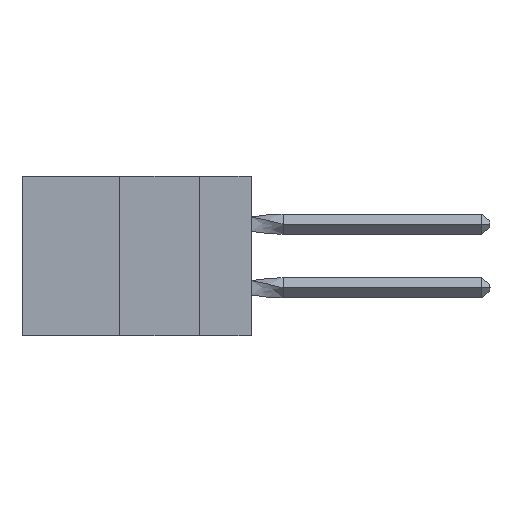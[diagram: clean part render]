
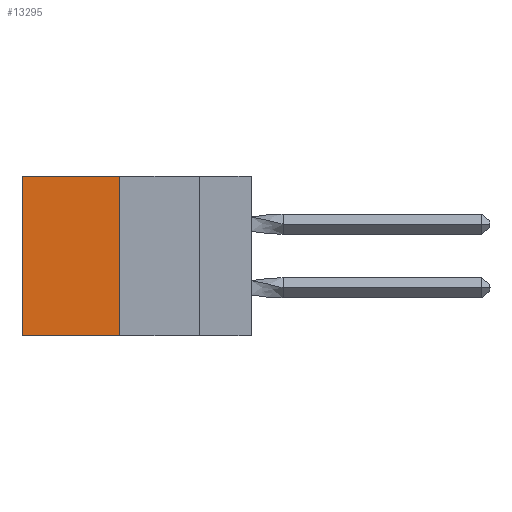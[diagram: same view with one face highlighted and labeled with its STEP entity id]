
A CAD part, left-side view. The second image highlights one B-rep face of the part: STEP entity #13295.
In plain terms, the highlighted planar face has unit normal (-1, 0, 0).
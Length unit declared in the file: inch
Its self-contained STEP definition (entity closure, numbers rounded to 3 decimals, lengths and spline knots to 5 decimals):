
#502 = CARTESIAN_POINT ( 'NONE',  ( 0.305, 0.72, 0. ) ) ;
#1578 = VERTEX_POINT ( 'NONE', #7610 ) ;
#1624 = DIRECTION ( 'NONE',  ( 0., 1., 0. ) ) ;
#2292 = DIRECTION ( 'NONE',  ( 1., 0., 0. ) ) ;
#2792 = CARTESIAN_POINT ( 'NONE',  ( 0.305, 0.413, -0.5 ) ) ;
#2944 = ORIENTED_EDGE ( 'NONE', *, *, #9007, .F. ) ;
#3227 = CARTESIAN_POINT ( 'NONE',  ( 0.305, 0.72, -0.5 ) ) ;
#3410 = VECTOR ( 'NONE', #1624, 39.37008 ) ;
#3446 = CARTESIAN_POINT ( 'NONE',  ( 0.305, 0.413, -0.5 ) ) ;
#4128 = FACE_OUTER_BOUND ( 'NONE', #6874, .T. ) ;
#4388 = DIRECTION ( 'NONE',  ( 0., 0., -1. ) ) ;
#5078 = VECTOR ( 'NONE', #4388, 39.37008 ) ;
#5505 = LINE ( 'NONE', #14696, #13486 ) ;
#5986 = CARTESIAN_POINT ( 'NONE',  ( 0.305, 0.72, -0.5 ) ) ;
#6098 = VERTEX_POINT ( 'NONE', #14415 ) ;
#6152 = LINE ( 'NONE', #7355, #3410 ) ;
#6251 = ORIENTED_EDGE ( 'NONE', *, *, #9287, .F. ) ;
#6668 = EDGE_CURVE ( 'NONE', #6098, #13045, #6152, .T. ) ;
#6874 = EDGE_LOOP ( 'NONE', ( #14839, #6251, #2944, #12947 ) ) ;
#6926 = DIRECTION ( 'NONE',  ( 0., 0., -1. ) ) ;
#7082 = PLANE ( 'NONE',  #9610 ) ;
#7355 = CARTESIAN_POINT ( 'NONE',  ( 0.305, 0.413, 0. ) ) ;
#7610 = CARTESIAN_POINT ( 'NONE',  ( 0.305, 0.413, -0.5 ) ) ;
#7823 = VERTEX_POINT ( 'NONE', #5986 ) ;
#7859 = VECTOR ( 'NONE', #13160, 39.37008 ) ;
#8211 = LINE ( 'NONE', #2792, #7859 ) ;
#9007 = EDGE_CURVE ( 'NONE', #6098, #1578, #5505, .T. ) ;
#9287 = EDGE_CURVE ( 'NONE', #1578, #7823, #8211, .T. ) ;
#9610 = AXIS2_PLACEMENT_3D ( 'NONE', #3446, #2292, #6926 ) ;
#9773 = LINE ( 'NONE', #3227, #5078 ) ;
#11011 = EDGE_CURVE ( 'NONE', #13045, #7823, #9773, .T. ) ;
#12655 = DIRECTION ( 'NONE',  ( 0., 0., -1. ) ) ;
#12947 = ORIENTED_EDGE ( 'NONE', *, *, #6668, .T. ) ;
#13045 = VERTEX_POINT ( 'NONE', #502 ) ;
#13160 = DIRECTION ( 'NONE',  ( 0., 1., 0. ) ) ;
#13295 = ADVANCED_FACE ( 'NONE', ( #4128 ), #7082, .F. ) ;
#13486 = VECTOR ( 'NONE', #12655, 39.37008 ) ;
#14415 = CARTESIAN_POINT ( 'NONE',  ( 0.305, 0.413, 0. ) ) ;
#14696 = CARTESIAN_POINT ( 'NONE',  ( 0.305, 0.413, -0.5 ) ) ;
#14839 = ORIENTED_EDGE ( 'NONE', *, *, #11011, .T. ) ;
